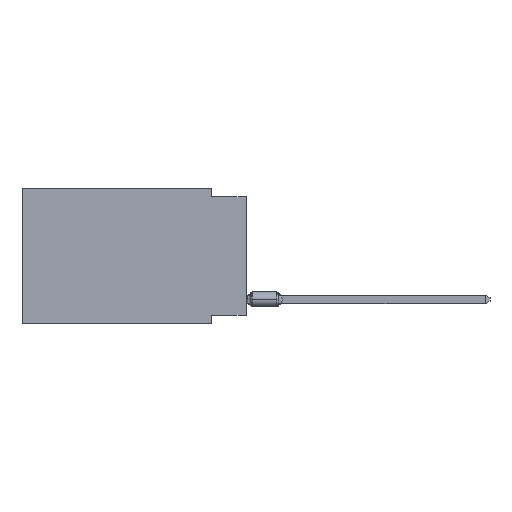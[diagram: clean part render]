
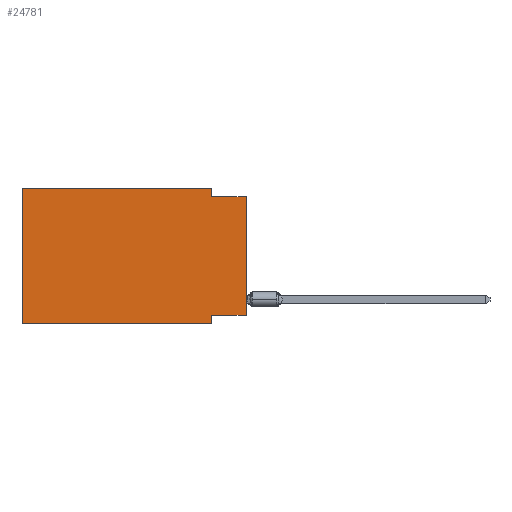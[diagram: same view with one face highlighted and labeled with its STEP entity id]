
A CAD part, left-side view. The second image highlights one B-rep face of the part: STEP entity #24781.
In plain terms, the highlighted planar face has unit normal (-1, 0, 0).
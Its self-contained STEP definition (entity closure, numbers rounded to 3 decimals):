
#962 = EDGE_CURVE ( 'NONE', #23792, #4495, #13761, .T. ) ;
#1146 = ORIENTED_EDGE ( 'NONE', *, *, #3972, .F. ) ;
#1543 = DIRECTION ( 'NONE',  ( 0., 0., -1. ) ) ;
#1783 = VECTOR ( 'NONE', #14193, 1000. ) ;
#1833 = ORIENTED_EDGE ( 'NONE', *, *, #962, .F. ) ;
#2123 = DIRECTION ( 'NONE',  ( 0., -1., 0. ) ) ;
#2619 = ORIENTED_EDGE ( 'NONE', *, *, #4045, .F. ) ;
#3062 = EDGE_CURVE ( 'NONE', #13288, #23792, #16739, .T. ) ;
#3972 = EDGE_CURVE ( 'NONE', #5947, #29450, #18519, .T. ) ;
#4045 = EDGE_CURVE ( 'NONE', #29649, #23073, #21126, .T. ) ;
#4495 = VERTEX_POINT ( 'NONE', #15839 ) ;
#4722 = DIRECTION ( 'NONE',  ( 0., -1., 0. ) ) ;
#5810 = ORIENTED_EDGE ( 'NONE', *, *, #26953, .T. ) ;
#5947 = VERTEX_POINT ( 'NONE', #8299 ) ;
#6197 = VECTOR ( 'NONE', #30251, 1000. ) ;
#7396 = CARTESIAN_POINT ( 'NONE',  ( 0., 0., 0. ) ) ;
#7853 = VECTOR ( 'NONE', #2123, 1000. ) ;
#7913 = CARTESIAN_POINT ( 'NONE',  ( 0., 16.383, 0. ) ) ;
#8299 = CARTESIAN_POINT ( 'NONE',  ( 0., 16.383, -9.906 ) ) ;
#8322 = LINE ( 'NONE', #15300, #27795 ) ;
#8538 = EDGE_CURVE ( 'NONE', #29450, #13288, #8322, .T. ) ;
#8873 = AXIS2_PLACEMENT_3D ( 'NONE', #10268, #24182, #26809 ) ;
#9379 = CARTESIAN_POINT ( 'NONE',  ( 0., 16.383, -9.906 ) ) ;
#9753 = ORIENTED_EDGE ( 'NONE', *, *, #8538, .F. ) ;
#10069 = DIRECTION ( 'NONE',  ( 0., 0., -1. ) ) ;
#10268 = CARTESIAN_POINT ( 'NONE',  ( 0., 16.383, 0. ) ) ;
#12234 = DIRECTION ( 'NONE',  ( 0., 0., 1. ) ) ;
#12405 = CARTESIAN_POINT ( 'NONE',  ( 0., 2.54, 0. ) ) ;
#13288 = VERTEX_POINT ( 'NONE', #27741 ) ;
#13424 = DIRECTION ( 'NONE',  ( 0., -1., 0. ) ) ;
#13761 = LINE ( 'NONE', #16380, #7853 ) ;
#13769 = EDGE_CURVE ( 'NONE', #29649, #4495, #26437, .T. ) ;
#13859 = VECTOR ( 'NONE', #4722, 1000. ) ;
#14193 = DIRECTION ( 'NONE',  ( 0., 0., 1. ) ) ;
#14752 = PLANE ( 'NONE',  #8873 ) ;
#15300 = CARTESIAN_POINT ( 'NONE',  ( 0., 16.383, 0. ) ) ;
#15839 = CARTESIAN_POINT ( 'NONE',  ( 0., 0., -0.635 ) ) ;
#16380 = CARTESIAN_POINT ( 'NONE',  ( 0., 0., -0.635 ) ) ;
#16739 = LINE ( 'NONE', #12405, #25458 ) ;
#16869 = CARTESIAN_POINT ( 'NONE',  ( 0., 0., -9.271 ) ) ;
#17676 = LINE ( 'NONE', #29853, #28429 ) ;
#18519 = LINE ( 'NONE', #18681, #1783 ) ;
#18681 = CARTESIAN_POINT ( 'NONE',  ( 0., 16.383, 0. ) ) ;
#19934 = ORIENTED_EDGE ( 'NONE', *, *, #13769, .T. ) ;
#20826 = CARTESIAN_POINT ( 'NONE',  ( 0., 0., -9.271 ) ) ;
#21126 = LINE ( 'NONE', #20826, #6197 ) ;
#21478 = CARTESIAN_POINT ( 'NONE',  ( 0., 2.54, -0.635 ) ) ;
#21606 = EDGE_CURVE ( 'NONE', #23073, #29338, #17676, .T. ) ;
#21925 = ORIENTED_EDGE ( 'NONE', *, *, #3062, .F. ) ;
#22643 = CARTESIAN_POINT ( 'NONE',  ( 0., 2.54, -9.271 ) ) ;
#23073 = VERTEX_POINT ( 'NONE', #22643 ) ;
#23792 = VERTEX_POINT ( 'NONE', #21478 ) ;
#24182 = DIRECTION ( 'NONE',  ( 1., 0., 0. ) ) ;
#24781 = ADVANCED_FACE ( 'NONE', ( #29293 ), #14752, .F. ) ;
#25458 = VECTOR ( 'NONE', #10069, 1000. ) ;
#26437 = LINE ( 'NONE', #7396, #30433 ) ;
#26809 = DIRECTION ( 'NONE',  ( 0., 0., -1. ) ) ;
#26953 = EDGE_CURVE ( 'NONE', #5947, #29338, #30584, .T. ) ;
#27741 = CARTESIAN_POINT ( 'NONE',  ( 0., 2.54, 0. ) ) ;
#27795 = VECTOR ( 'NONE', #13424, 1000. ) ;
#28429 = VECTOR ( 'NONE', #1543, 1000. ) ;
#28516 = CARTESIAN_POINT ( 'NONE',  ( 0., 2.54, -9.906 ) ) ;
#29222 = ORIENTED_EDGE ( 'NONE', *, *, #21606, .F. ) ;
#29293 = FACE_OUTER_BOUND ( 'NONE', #30311, .T. ) ;
#29338 = VERTEX_POINT ( 'NONE', #28516 ) ;
#29450 = VERTEX_POINT ( 'NONE', #7913 ) ;
#29649 = VERTEX_POINT ( 'NONE', #16869 ) ;
#29853 = CARTESIAN_POINT ( 'NONE',  ( 0., 2.54, -9.906 ) ) ;
#30251 = DIRECTION ( 'NONE',  ( 0., 1., 0. ) ) ;
#30311 = EDGE_LOOP ( 'NONE', ( #19934, #1833, #21925, #9753, #1146, #5810, #29222, #2619 ) ) ;
#30433 = VECTOR ( 'NONE', #12234, 1000. ) ;
#30584 = LINE ( 'NONE', #9379, #13859 ) ;
